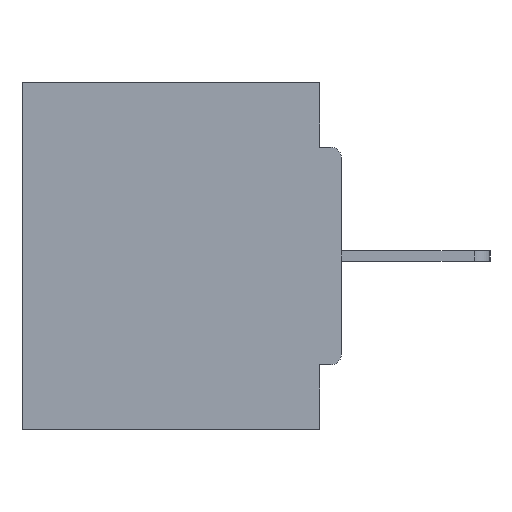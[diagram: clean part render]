
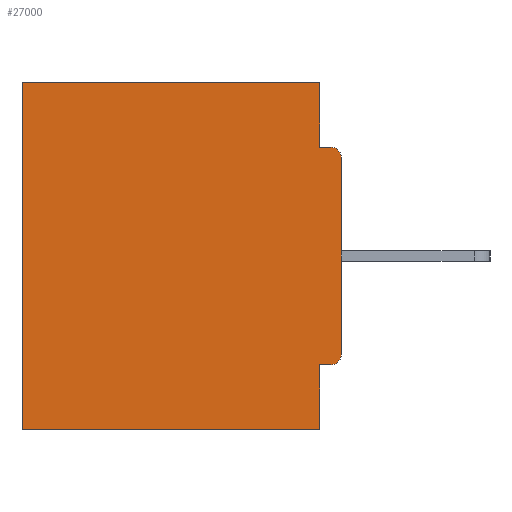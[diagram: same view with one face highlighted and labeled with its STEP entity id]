
A CAD part, left-side view. The second image highlights one B-rep face of the part: STEP entity #27000.
In plain terms, the highlighted planar face has unit normal (-1, 0, 0).
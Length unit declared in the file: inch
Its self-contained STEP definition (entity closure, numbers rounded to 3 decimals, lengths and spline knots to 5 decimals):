
#327 = CARTESIAN_POINT ( 'NONE',  ( 0.298, 0.46, 0. ) ) ;
#464 = VERTEX_POINT ( 'NONE', #6820 ) ;
#596 = VERTEX_POINT ( 'NONE', #18794 ) ;
#1231 = PLANE ( 'NONE',  #9295 ) ;
#1948 = DIRECTION ( 'NONE',  ( 0., 1., 0. ) ) ;
#2250 = VECTOR ( 'NONE', #11112, 39.37008 ) ;
#2358 = CARTESIAN_POINT ( 'NONE',  ( 0.298, 0., 0. ) ) ;
#2382 = EDGE_LOOP ( 'NONE', ( #10139, #24507, #6968, #4121, #3079, #22942, #17675, #11124, #24252, #25606 ) ) ;
#2766 = EDGE_CURVE ( 'NONE', #26992, #17272, #22595, .T. ) ;
#3079 = ORIENTED_EDGE ( 'NONE', *, *, #4375, .T. ) ;
#3551 = LINE ( 'NONE', #6050, #18197 ) ;
#4121 = ORIENTED_EDGE ( 'NONE', *, *, #2766, .T. ) ;
#4375 = EDGE_CURVE ( 'NONE', #17272, #17007, #7232, .T. ) ;
#5277 = DIRECTION ( 'NONE',  ( 0., 1., 0. ) ) ;
#6050 = CARTESIAN_POINT ( 'NONE',  ( 0.298, 0., -0.0935 ) ) ;
#6405 = EDGE_CURVE ( 'NONE', #7913, #7549, #8684, .T. ) ;
#6466 = DIRECTION ( 'NONE',  ( 0., 0., -1. ) ) ;
#6820 = CARTESIAN_POINT ( 'NONE',  ( 0.298, 0.031, -0.5 ) ) ;
#6968 = ORIENTED_EDGE ( 'NONE', *, *, #7279, .F. ) ;
#7018 = VERTEX_POINT ( 'NONE', #12711 ) ;
#7232 = LINE ( 'NONE', #327, #23918 ) ;
#7279 = EDGE_CURVE ( 'NONE', #26992, #7018, #27485, .T. ) ;
#7549 = VERTEX_POINT ( 'NONE', #8690 ) ;
#7913 = VERTEX_POINT ( 'NONE', #26119 ) ;
#7936 = DIRECTION ( 'NONE',  ( 0., 0., -1. ) ) ;
#8072 = DIRECTION ( 'NONE',  ( -1., 0., 0. ) ) ;
#8155 = VECTOR ( 'NONE', #6466, 39.37008 ) ;
#8684 = LINE ( 'NONE', #28494, #8155 ) ;
#8690 = CARTESIAN_POINT ( 'NONE',  ( 0.298, 0., -0.3915 ) ) ;
#9295 = AXIS2_PLACEMENT_3D ( 'NONE', #12590, #21169, #28275 ) ;
#9933 = FACE_OUTER_BOUND ( 'NONE', #2382, .T. ) ;
#10139 = ORIENTED_EDGE ( 'NONE', *, *, #20322, .T. ) ;
#10808 = VECTOR ( 'NONE', #1948, 39.37008 ) ;
#11112 = DIRECTION ( 'NONE',  ( 0., 1., 0. ) ) ;
#11124 = ORIENTED_EDGE ( 'NONE', *, *, #20053, .F. ) ;
#11244 = CARTESIAN_POINT ( 'NONE',  ( 0.298, 0., -0.4065 ) ) ;
#11542 = LINE ( 'NONE', #22334, #2250 ) ;
#12294 = CARTESIAN_POINT ( 'NONE',  ( 0.298, 0.015, -0.0935 ) ) ;
#12473 = VECTOR ( 'NONE', #16321, 39.37008 ) ;
#12590 = CARTESIAN_POINT ( 'NONE',  ( 0.298, 0., 0. ) ) ;
#12711 = CARTESIAN_POINT ( 'NONE',  ( 0.298, 0.031, -0.0935 ) ) ;
#14172 = CARTESIAN_POINT ( 'NONE',  ( 0.298, 0.46, 0. ) ) ;
#15031 = CARTESIAN_POINT ( 'NONE',  ( 0.298, 0.015, -0.3915 ) ) ;
#15080 = LINE ( 'NONE', #11244, #10808 ) ;
#15393 = CIRCLE ( 'NONE', #20106, 0.015 ) ;
#16321 = DIRECTION ( 'NONE',  ( 0., 0., -1. ) ) ;
#16823 = DIRECTION ( 'NONE',  ( -1., 0., 0. ) ) ;
#16946 = CIRCLE ( 'NONE', #24486, 0.015 ) ;
#17007 = VERTEX_POINT ( 'NONE', #25727 ) ;
#17272 = VERTEX_POINT ( 'NONE', #14172 ) ;
#17409 = VECTOR ( 'NONE', #5277, 39.37008 ) ;
#17675 = ORIENTED_EDGE ( 'NONE', *, *, #28649, .F. ) ;
#18167 = CARTESIAN_POINT ( 'NONE',  ( 0.298, 0.031, -0.5 ) ) ;
#18197 = VECTOR ( 'NONE', #21572, 39.37008 ) ;
#18533 = VERTEX_POINT ( 'NONE', #12294 ) ;
#18794 = CARTESIAN_POINT ( 'NONE',  ( 0.298, 0.015, -0.4065 ) ) ;
#20053 = EDGE_CURVE ( 'NONE', #596, #21743, #15080, .T. ) ;
#20106 = AXIS2_PLACEMENT_3D ( 'NONE', #15031, #8072, #7936 ) ;
#20322 = EDGE_CURVE ( 'NONE', #7913, #18533, #16946, .T. ) ;
#21169 = DIRECTION ( 'NONE',  ( 1., 0., 0. ) ) ;
#21572 = DIRECTION ( 'NONE',  ( 0., -1., 0. ) ) ;
#21743 = VERTEX_POINT ( 'NONE', #26079 ) ;
#22334 = CARTESIAN_POINT ( 'NONE',  ( 0.298, 0., -0.5 ) ) ;
#22595 = LINE ( 'NONE', #2358, #17409 ) ;
#22807 = CARTESIAN_POINT ( 'NONE',  ( 0.298, 0.031, 0. ) ) ;
#22942 = ORIENTED_EDGE ( 'NONE', *, *, #27315, .F. ) ;
#23121 = CARTESIAN_POINT ( 'NONE',  ( 0.298, 0.031, -0.5 ) ) ;
#23478 = DIRECTION ( 'NONE',  ( 0., 0., -1. ) ) ;
#23918 = VECTOR ( 'NONE', #24845, 39.37008 ) ;
#23926 = CARTESIAN_POINT ( 'NONE',  ( 0.298, 0.015, -0.1085 ) ) ;
#24040 = EDGE_CURVE ( 'NONE', #7018, #18533, #3551, .T. ) ;
#24252 = ORIENTED_EDGE ( 'NONE', *, *, #26354, .T. ) ;
#24486 = AXIS2_PLACEMENT_3D ( 'NONE', #23926, #16823, #23478 ) ;
#24507 = ORIENTED_EDGE ( 'NONE', *, *, #24040, .F. ) ;
#24845 = DIRECTION ( 'NONE',  ( 0., 0., -1. ) ) ;
#25375 = VECTOR ( 'NONE', #27637, 39.37008 ) ;
#25606 = ORIENTED_EDGE ( 'NONE', *, *, #6405, .F. ) ;
#25727 = CARTESIAN_POINT ( 'NONE',  ( 0.298, 0.46, -0.5 ) ) ;
#26079 = CARTESIAN_POINT ( 'NONE',  ( 0.298, 0.031, -0.4065 ) ) ;
#26119 = CARTESIAN_POINT ( 'NONE',  ( 0.298, 0., -0.1085 ) ) ;
#26354 = EDGE_CURVE ( 'NONE', #596, #7549, #15393, .T. ) ;
#26992 = VERTEX_POINT ( 'NONE', #22807 ) ;
#27000 = ADVANCED_FACE ( 'NONE', ( #9933 ), #1231, .F. ) ;
#27315 = EDGE_CURVE ( 'NONE', #464, #17007, #11542, .T. ) ;
#27485 = LINE ( 'NONE', #18167, #25375 ) ;
#27570 = LINE ( 'NONE', #23121, #12473 ) ;
#27637 = DIRECTION ( 'NONE',  ( 0., 0., -1. ) ) ;
#28275 = DIRECTION ( 'NONE',  ( 0., 0., -1. ) ) ;
#28494 = CARTESIAN_POINT ( 'NONE',  ( 0.298, 0., 0. ) ) ;
#28649 = EDGE_CURVE ( 'NONE', #21743, #464, #27570, .T. ) ;
